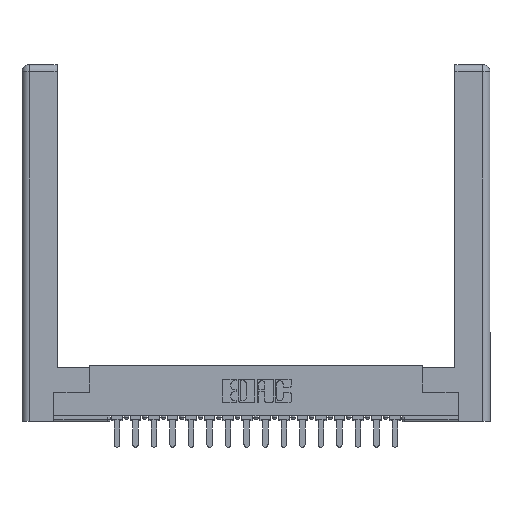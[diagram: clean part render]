
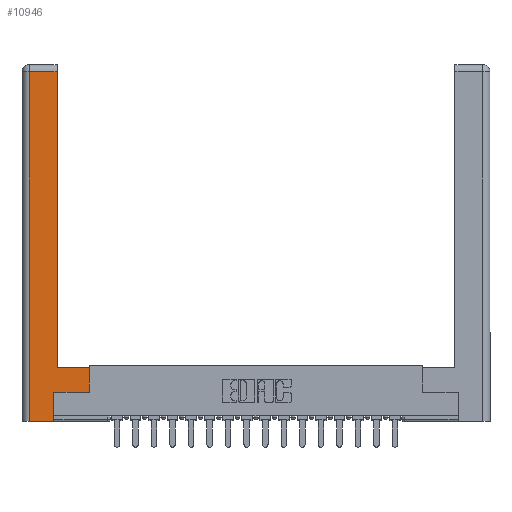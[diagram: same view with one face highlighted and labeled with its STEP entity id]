
A CAD part, top view. The second image highlights one B-rep face of the part: STEP entity #10946.
In plain terms, the highlighted planar face has unit normal (0, 0, 1).
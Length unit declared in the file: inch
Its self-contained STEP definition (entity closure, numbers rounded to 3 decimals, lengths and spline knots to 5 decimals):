
#151 = FACE_OUTER_BOUND ( 'NONE', #5148, .T. ) ;
#404 = ORIENTED_EDGE ( 'NONE', *, *, #13196, .T. ) ;
#487 = CARTESIAN_POINT ( 'NONE',  ( 0.565, 0.245, 0. ) ) ;
#503 = ORIENTED_EDGE ( 'NONE', *, *, #5253, .T. ) ;
#1582 = ORIENTED_EDGE ( 'NONE', *, *, #8364, .T. ) ;
#1601 = VERTEX_POINT ( 'NONE', #17260 ) ;
#1614 = VERTEX_POINT ( 'NONE', #6314 ) ;
#1942 = CARTESIAN_POINT ( 'NONE',  ( 0.295, 0.45, 0. ) ) ;
#2258 = EDGE_CURVE ( 'NONE', #14255, #5746, #2338, .T. ) ;
#2338 = LINE ( 'NONE', #487, #6523 ) ;
#2968 = VECTOR ( 'NONE', #18826, 39.37008 ) ;
#3044 = VERTEX_POINT ( 'NONE', #13592 ) ;
#3690 = EDGE_CURVE ( 'NONE', #5746, #3044, #19851, .T. ) ;
#3812 = ORIENTED_EDGE ( 'NONE', *, *, #16922, .T. ) ;
#3831 = EDGE_CURVE ( 'NONE', #11578, #12462, #18172, .T. ) ;
#4186 = VECTOR ( 'NONE', #20100, 39.37008 ) ;
#4795 = DIRECTION ( 'NONE',  ( -1., 0., 0. ) ) ;
#5148 = EDGE_LOOP ( 'NONE', ( #404, #503, #14259, #3812, #16518, #9781, #20135, #1582 ) ) ;
#5253 = EDGE_CURVE ( 'NONE', #1614, #11578, #12010, .T. ) ;
#5746 = VERTEX_POINT ( 'NONE', #8688 ) ;
#6161 = CARTESIAN_POINT ( 'NONE',  ( 0.265, 0.245, 0. ) ) ;
#6314 = CARTESIAN_POINT ( 'NONE',  ( 0.295, 2.94, 0. ) ) ;
#6523 = VECTOR ( 'NONE', #6880, 39.37008 ) ;
#6880 = DIRECTION ( 'NONE',  ( 1., 0., 0. ) ) ;
#6939 = LINE ( 'NONE', #17501, #14508 ) ;
#7835 = PLANE ( 'NONE',  #9744 ) ;
#8031 = CARTESIAN_POINT ( 'NONE',  ( 0.0615, 0., 0. ) ) ;
#8364 = EDGE_CURVE ( 'NONE', #3044, #1601, #8841, .T. ) ;
#8688 = CARTESIAN_POINT ( 'NONE',  ( 0.565, 0.245, 0. ) ) ;
#8841 = LINE ( 'NONE', #1942, #12512 ) ;
#9574 = DIRECTION ( 'NONE',  ( 1., 0., 0. ) ) ;
#9744 = AXIS2_PLACEMENT_3D ( 'NONE', #18754, #18828, #4795 ) ;
#9781 = ORIENTED_EDGE ( 'NONE', *, *, #2258, .T. ) ;
#10553 = LINE ( 'NONE', #6161, #11544 ) ;
#10946 = ADVANCED_FACE ( 'NONE', ( #151 ), #7835, .F. ) ;
#11544 = VECTOR ( 'NONE', #20206, 39.37008 ) ;
#11578 = VERTEX_POINT ( 'NONE', #13469 ) ;
#12010 = LINE ( 'NONE', #14742, #14445 ) ;
#12267 = CARTESIAN_POINT ( 'NONE',  ( 0.565, 0.45, 0. ) ) ;
#12462 = VERTEX_POINT ( 'NONE', #8031 ) ;
#12512 = VECTOR ( 'NONE', #14468, 39.37008 ) ;
#13003 = CARTESIAN_POINT ( 'NONE',  ( 0.295, 3., 0. ) ) ;
#13196 = EDGE_CURVE ( 'NONE', #1601, #1614, #17090, .T. ) ;
#13469 = CARTESIAN_POINT ( 'NONE',  ( 0.0615, 2.94, 0. ) ) ;
#13592 = CARTESIAN_POINT ( 'NONE',  ( 0.565, 0.45, 0. ) ) ;
#14239 = CARTESIAN_POINT ( 'NONE',  ( 0.0615, 0., 0. ) ) ;
#14255 = VERTEX_POINT ( 'NONE', #15251 ) ;
#14259 = ORIENTED_EDGE ( 'NONE', *, *, #3831, .T. ) ;
#14445 = VECTOR ( 'NONE', #16449, 39.37008 ) ;
#14468 = DIRECTION ( 'NONE',  ( -1., 0., 0. ) ) ;
#14508 = VECTOR ( 'NONE', #9574, 39.37008 ) ;
#14742 = CARTESIAN_POINT ( 'NONE',  ( 0.0615, 2.94, 0. ) ) ;
#14796 = CARTESIAN_POINT ( 'NONE',  ( 0.265, 0., 0. ) ) ;
#15251 = CARTESIAN_POINT ( 'NONE',  ( 0.265, 0.245, 0. ) ) ;
#16141 = DIRECTION ( 'NONE',  ( 0., 1., 0. ) ) ;
#16449 = DIRECTION ( 'NONE',  ( -1., 0., 0. ) ) ;
#16518 = ORIENTED_EDGE ( 'NONE', *, *, #18153, .T. ) ;
#16922 = EDGE_CURVE ( 'NONE', #12462, #19117, #6939, .T. ) ;
#17090 = LINE ( 'NONE', #13003, #18551 ) ;
#17260 = CARTESIAN_POINT ( 'NONE',  ( 0.295, 0.45, 0. ) ) ;
#17501 = CARTESIAN_POINT ( 'NONE',  ( 0.265, 0., 0. ) ) ;
#18153 = EDGE_CURVE ( 'NONE', #19117, #14255, #10553, .T. ) ;
#18172 = LINE ( 'NONE', #14239, #2968 ) ;
#18551 = VECTOR ( 'NONE', #16141, 39.37008 ) ;
#18754 = CARTESIAN_POINT ( 'NONE',  ( 0., 0., 0. ) ) ;
#18826 = DIRECTION ( 'NONE',  ( 0., -1., 0. ) ) ;
#18828 = DIRECTION ( 'NONE',  ( 0., 0., -1. ) ) ;
#19117 = VERTEX_POINT ( 'NONE', #14796 ) ;
#19851 = LINE ( 'NONE', #12267, #4186 ) ;
#20100 = DIRECTION ( 'NONE',  ( 0., 1., 0. ) ) ;
#20135 = ORIENTED_EDGE ( 'NONE', *, *, #3690, .T. ) ;
#20206 = DIRECTION ( 'NONE',  ( 0., 1., 0. ) ) ;
